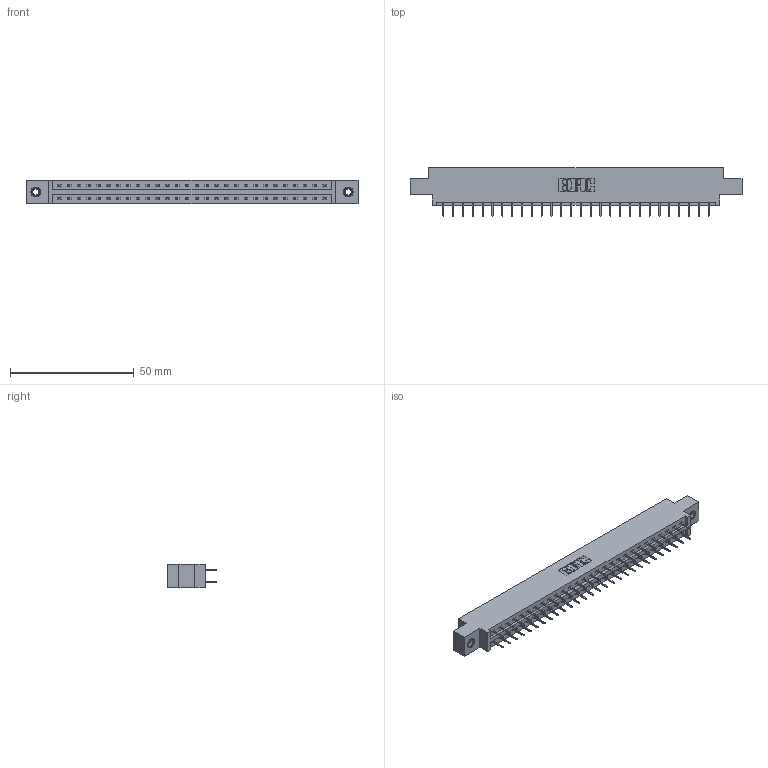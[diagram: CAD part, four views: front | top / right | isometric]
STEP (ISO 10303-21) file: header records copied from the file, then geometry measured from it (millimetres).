
FILE_DESCRIPTION (( 'STEP AP203' ), '1' );
FILE_NAME ('387-056-524-807.STEP', '2018-09-20T23:39:16', ( '' ), ( '' ), 'SwSTEP 2.0', 'SolidWorks 2016', '' );
FILE_SCHEMA (( 'CONFIG_CONTROL_DESIGN' ));
Length unit declared in the file: inch
Products named in the file (4): 345-292-001_345-293-124; 345-250-001_345-250-005-103; 387-056-524-807; 337 Part_0.170 Offset - 0.156 Dia-TI
Assembly tree (59 placements, depth 2):
  387-056-524-807
    337 Part_0.170 Offset - 0.156 Dia-TI
    345-292-001_345-293-124  x56
    345-250-001_345-250-005-103  x2
Bounding box: 133.96 x 19.69 x 9.4 mm (x, y, z)
Volume: 13715.6 mm3; surface area: 15250.8 mm2
Topology: 59 solids, 59 shells, 3426 faces, 9699 edges, 6234 vertices
Faces by surface type: plane 2570, cylinder 840, cone 12, torus 4
Entity records: 24912 total; most frequent: CARTESIAN_POINT 4189, ORIENTED_EDGE 4118, DIRECTION 3621, EDGE_CURVE 2059, LINE 1915, VECTOR 1915, VERTEX_POINT 1364, AXIS2_PLACEMENT_3D 853
